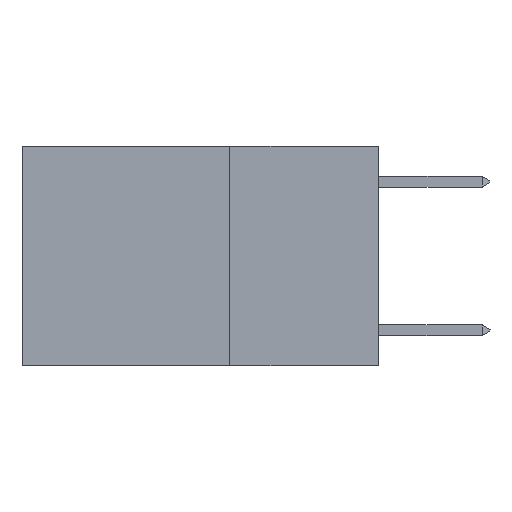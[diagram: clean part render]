
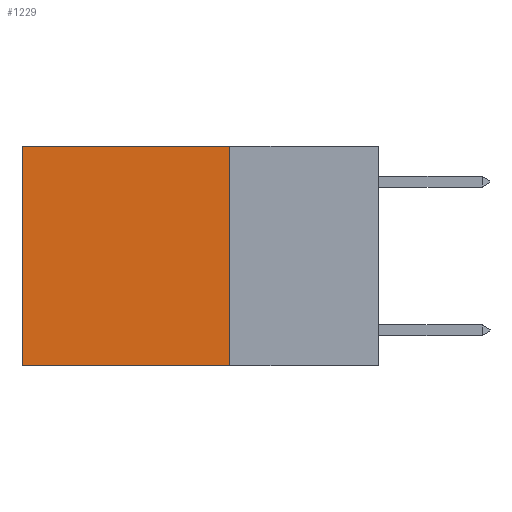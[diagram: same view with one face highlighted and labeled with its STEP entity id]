
A CAD part, left-side view. The second image highlights one B-rep face of the part: STEP entity #1229.
In plain terms, the highlighted planar face has unit normal (-1, 0, 0).
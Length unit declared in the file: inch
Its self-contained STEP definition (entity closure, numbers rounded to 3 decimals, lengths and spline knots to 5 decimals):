
#22 = VERTEX_POINT ( 'NONE', #8934 ) ;
#184 = VECTOR ( 'NONE', #7703, 39.37008 ) ;
#455 = LINE ( 'NONE', #8456, #184 ) ;
#879 = CARTESIAN_POINT ( 'NONE',  ( 0.2625, 0.25, 0. ) ) ;
#1229 = ADVANCED_FACE ( 'NONE', ( #2957 ), #8863, .F. ) ;
#1347 = EDGE_CURVE ( 'NONE', #3443, #6366, #9161, .T. ) ;
#1948 = CARTESIAN_POINT ( 'NONE',  ( 0.2625, 0.25, -0.37 ) ) ;
#2393 = ORIENTED_EDGE ( 'NONE', *, *, #9182, .F. ) ;
#2550 = DIRECTION ( 'NONE',  ( 0., 0., -1. ) ) ;
#2600 = EDGE_CURVE ( 'NONE', #6366, #22, #455, .T. ) ;
#2732 = DIRECTION ( 'NONE',  ( 0., 1., 0. ) ) ;
#2957 = FACE_OUTER_BOUND ( 'NONE', #6273, .T. ) ;
#3443 = VERTEX_POINT ( 'NONE', #6367 ) ;
#3578 = ORIENTED_EDGE ( 'NONE', *, *, #2600, .T. ) ;
#3608 = ORIENTED_EDGE ( 'NONE', *, *, #6702, .F. ) ;
#3975 = AXIS2_PLACEMENT_3D ( 'NONE', #879, #5261, #2550 ) ;
#4012 = CARTESIAN_POINT ( 'NONE',  ( 0.2625, 0.25, 0. ) ) ;
#4374 = VERTEX_POINT ( 'NONE', #6518 ) ;
#4748 = DIRECTION ( 'NONE',  ( 0., 0., -1. ) ) ;
#5113 = LINE ( 'NONE', #1948, #8814 ) ;
#5261 = DIRECTION ( 'NONE',  ( 1., 0., 0. ) ) ;
#5282 = CARTESIAN_POINT ( 'NONE',  ( 0.2625, 0.6, 0. ) ) ;
#5520 = VECTOR ( 'NONE', #4748, 39.37008 ) ;
#6273 = EDGE_LOOP ( 'NONE', ( #3578, #3608, #2393, #9169 ) ) ;
#6366 = VERTEX_POINT ( 'NONE', #5282 ) ;
#6367 = CARTESIAN_POINT ( 'NONE',  ( 0.2625, 0.25, 0. ) ) ;
#6518 = CARTESIAN_POINT ( 'NONE',  ( 0.2625, 0.25, -0.37 ) ) ;
#6702 = EDGE_CURVE ( 'NONE', #4374, #22, #5113, .T. ) ;
#7200 = VECTOR ( 'NONE', #8064, 39.37008 ) ;
#7703 = DIRECTION ( 'NONE',  ( 0., 0., -1. ) ) ;
#8064 = DIRECTION ( 'NONE',  ( 0., 1., 0. ) ) ;
#8456 = CARTESIAN_POINT ( 'NONE',  ( 0.2625, 0.6, 0. ) ) ;
#8814 = VECTOR ( 'NONE', #2732, 39.37008 ) ;
#8863 = PLANE ( 'NONE',  #3975 ) ;
#8934 = CARTESIAN_POINT ( 'NONE',  ( 0.2625, 0.6, -0.37 ) ) ;
#9161 = LINE ( 'NONE', #9526, #7200 ) ;
#9169 = ORIENTED_EDGE ( 'NONE', *, *, #1347, .T. ) ;
#9182 = EDGE_CURVE ( 'NONE', #3443, #4374, #9460, .T. ) ;
#9460 = LINE ( 'NONE', #4012, #5520 ) ;
#9526 = CARTESIAN_POINT ( 'NONE',  ( 0.2625, 0.25, 0. ) ) ;
